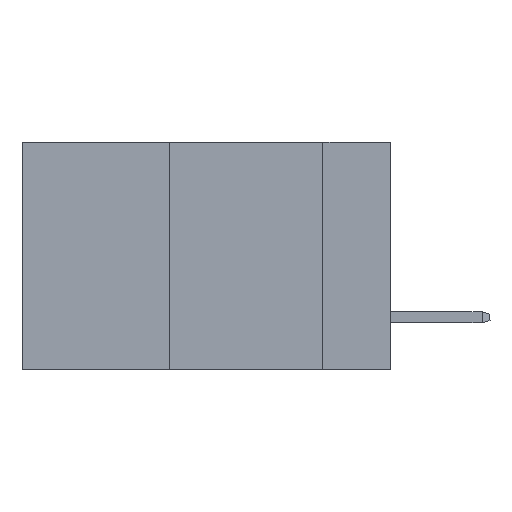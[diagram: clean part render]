
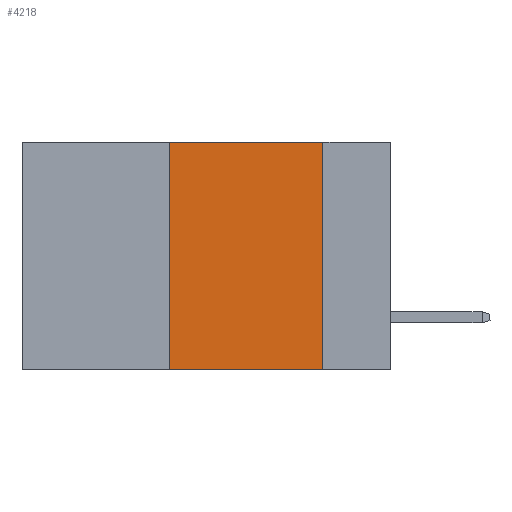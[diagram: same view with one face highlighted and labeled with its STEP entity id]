
A CAD part, left-side view. The second image highlights one B-rep face of the part: STEP entity #4218.
In plain terms, the highlighted planar face has unit normal (-1, 0, 0).
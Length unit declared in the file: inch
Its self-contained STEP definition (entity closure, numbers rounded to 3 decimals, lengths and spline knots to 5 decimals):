
#174 = VECTOR ( 'NONE', #7495, 39.37008 ) ;
#2205 = CARTESIAN_POINT ( 'NONE',  ( 0., 0.11, 0. ) ) ;
#2513 = CARTESIAN_POINT ( 'NONE',  ( 0., 0.36, 0. ) ) ;
#4218 = ADVANCED_FACE ( 'NONE', ( #12437 ), #20716, .F. ) ;
#4976 = CARTESIAN_POINT ( 'NONE',  ( 0., 0.6, 0. ) ) ;
#7091 = ORIENTED_EDGE ( 'NONE', *, *, #8237, .F. ) ;
#7257 = ORIENTED_EDGE ( 'NONE', *, *, #12198, .F. ) ;
#7495 = DIRECTION ( 'NONE',  ( 0., -1., 0. ) ) ;
#7811 = ORIENTED_EDGE ( 'NONE', *, *, #32107, .F. ) ;
#8020 = ORIENTED_EDGE ( 'NONE', *, *, #23823, .T. ) ;
#8237 = EDGE_CURVE ( 'NONE', #10975, #23416, #9050, .T. ) ;
#8281 = VECTOR ( 'NONE', #11215, 39.37008 ) ;
#8458 = VERTEX_POINT ( 'NONE', #27613 ) ;
#8707 = CARTESIAN_POINT ( 'NONE',  ( 0., 0.36, 0. ) ) ;
#9050 = LINE ( 'NONE', #9389, #21491 ) ;
#9389 = CARTESIAN_POINT ( 'NONE',  ( 0., 0.11, 0. ) ) ;
#10930 = CARTESIAN_POINT ( 'NONE',  ( 0., 0.6, 0. ) ) ;
#10975 = VERTEX_POINT ( 'NONE', #2205 ) ;
#11215 = DIRECTION ( 'NONE',  ( 0., 0., 1. ) ) ;
#11914 = DIRECTION ( 'NONE',  ( 0., 0., -1. ) ) ;
#12198 = EDGE_CURVE ( 'NONE', #21148, #10975, #13714, .T. ) ;
#12305 = CARTESIAN_POINT ( 'NONE',  ( 0., 0.6, -0.37 ) ) ;
#12437 = FACE_OUTER_BOUND ( 'NONE', #23139, .T. ) ;
#13477 = DIRECTION ( 'NONE',  ( 1., 0., 0. ) ) ;
#13714 = LINE ( 'NONE', #4976, #174 ) ;
#14351 = VECTOR ( 'NONE', #14841, 39.37008 ) ;
#14841 = DIRECTION ( 'NONE',  ( 0., -1., 0. ) ) ;
#20716 = PLANE ( 'NONE',  #29893 ) ;
#21148 = VERTEX_POINT ( 'NONE', #2513 ) ;
#21491 = VECTOR ( 'NONE', #11914, 39.37008 ) ;
#23128 = CARTESIAN_POINT ( 'NONE',  ( 0., 0.11, -0.37 ) ) ;
#23139 = EDGE_LOOP ( 'NONE', ( #7091, #7257, #7811, #8020 ) ) ;
#23416 = VERTEX_POINT ( 'NONE', #23128 ) ;
#23823 = EDGE_CURVE ( 'NONE', #8458, #23416, #27494, .T. ) ;
#27494 = LINE ( 'NONE', #12305, #14351 ) ;
#27613 = CARTESIAN_POINT ( 'NONE',  ( 0., 0.36, -0.37 ) ) ;
#28085 = LINE ( 'NONE', #8707, #8281 ) ;
#29893 = AXIS2_PLACEMENT_3D ( 'NONE', #10930, #13477, #30726 ) ;
#30726 = DIRECTION ( 'NONE',  ( 0., 0., -1. ) ) ;
#32107 = EDGE_CURVE ( 'NONE', #8458, #21148, #28085, .T. ) ;
